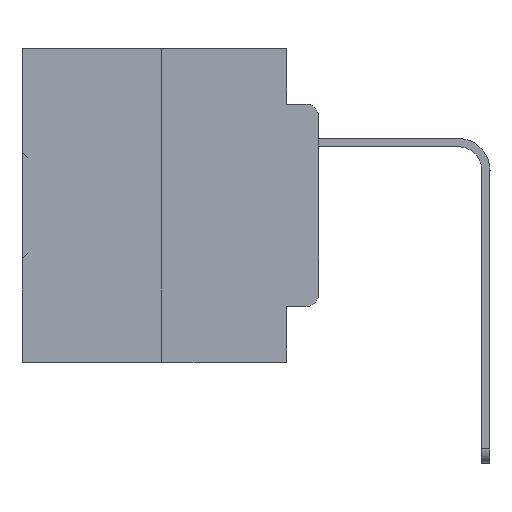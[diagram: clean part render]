
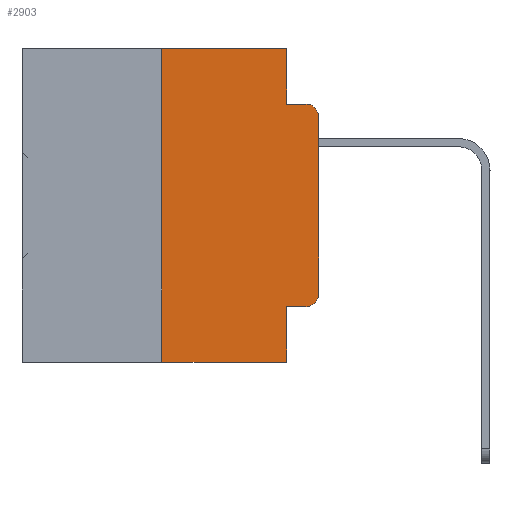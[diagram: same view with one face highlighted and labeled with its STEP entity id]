
A CAD part, left-side view. The second image highlights one B-rep face of the part: STEP entity #2903.
In plain terms, the highlighted planar face has unit normal (-1, 0, 0).
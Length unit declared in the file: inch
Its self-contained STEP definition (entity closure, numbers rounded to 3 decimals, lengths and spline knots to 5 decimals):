
#876 = EDGE_LOOP ( 'NONE', ( #3485, #27984, #14469, #26776, #28233, #36479, #4649, #27697, #25690, #18852 ) ) ;
#1336 = DIRECTION ( 'NONE',  ( 0., 0., -1. ) ) ;
#1850 = CARTESIAN_POINT ( 'NONE',  ( 0., 0.051, -0.4115 ) ) ;
#2461 = EDGE_CURVE ( 'NONE', #5087, #25818, #3342, .T. ) ;
#2837 = DIRECTION ( 'NONE',  ( 0., -1., 0. ) ) ;
#2903 = ADVANCED_FACE ( 'NONE', ( #31973 ), #5675, .F. ) ;
#3047 = DIRECTION ( 'NONE',  ( 0., 0., -1. ) ) ;
#3148 = VERTEX_POINT ( 'NONE', #23831 ) ;
#3251 = CIRCLE ( 'NONE', #27293, 0.02 ) ;
#3342 = LINE ( 'NONE', #25130, #12143 ) ;
#3485 = ORIENTED_EDGE ( 'NONE', *, *, #24115, .T. ) ;
#4204 = DIRECTION ( 'NONE',  ( 0., 0., 1. ) ) ;
#4649 = ORIENTED_EDGE ( 'NONE', *, *, #34257, .T. ) ;
#5087 = VERTEX_POINT ( 'NONE', #1850 ) ;
#5675 = PLANE ( 'NONE',  #17925 ) ;
#6218 = EDGE_CURVE ( 'NONE', #18391, #14889, #28655, .T. ) ;
#6763 = EDGE_CURVE ( 'NONE', #32839, #18391, #25930, .T. ) ;
#7319 = AXIS2_PLACEMENT_3D ( 'NONE', #21485, #21722, #10677 ) ;
#7865 = LINE ( 'NONE', #14119, #29493 ) ;
#9193 = EDGE_CURVE ( 'NONE', #25818, #26109, #3251, .T. ) ;
#9205 = VECTOR ( 'NONE', #1336, 39.37008 ) ;
#9571 = VECTOR ( 'NONE', #4204, 39.37008 ) ;
#9759 = CARTESIAN_POINT ( 'NONE',  ( 0., 0., 0. ) ) ;
#10613 = LINE ( 'NONE', #32290, #28263 ) ;
#10677 = DIRECTION ( 'NONE',  ( 0., 0., -1. ) ) ;
#11140 = CARTESIAN_POINT ( 'NONE',  ( 0., 0.02, -0.4115 ) ) ;
#12143 = VECTOR ( 'NONE', #2837, 39.37008 ) ;
#12409 = EDGE_CURVE ( 'NONE', #31313, #32839, #15794, .T. ) ;
#12755 = EDGE_CURVE ( 'NONE', #17602, #14889, #33425, .T. ) ;
#13996 = CARTESIAN_POINT ( 'NONE',  ( 0., 0.25, -0.5 ) ) ;
#14049 = CARTESIAN_POINT ( 'NONE',  ( 0., 0.473, 0. ) ) ;
#14119 = CARTESIAN_POINT ( 'NONE',  ( 0., 0.473, -0.5 ) ) ;
#14469 = ORIENTED_EDGE ( 'NONE', *, *, #6218, .F. ) ;
#14889 = VERTEX_POINT ( 'NONE', #31507 ) ;
#14898 = VECTOR ( 'NONE', #32012, 39.37008 ) ;
#15393 = CARTESIAN_POINT ( 'NONE',  ( 0., 0.051, 0. ) ) ;
#15545 = CARTESIAN_POINT ( 'NONE',  ( 0., 0.02, -0.3915 ) ) ;
#15794 = LINE ( 'NONE', #33511, #14898 ) ;
#16038 = CARTESIAN_POINT ( 'NONE',  ( 0., 0., -0.1085 ) ) ;
#16586 = DIRECTION ( 'NONE',  ( 0., -1., 0. ) ) ;
#17551 = EDGE_CURVE ( 'NONE', #21590, #31313, #10613, .T. ) ;
#17602 = VERTEX_POINT ( 'NONE', #16038 ) ;
#17925 = AXIS2_PLACEMENT_3D ( 'NONE', #14049, #25697, #3047 ) ;
#18391 = VERTEX_POINT ( 'NONE', #32585 ) ;
#18852 = ORIENTED_EDGE ( 'NONE', *, *, #9193, .T. ) ;
#19684 = LINE ( 'NONE', #9759, #9571 ) ;
#20548 = CARTESIAN_POINT ( 'NONE',  ( 0., 0., -0.3915 ) ) ;
#21032 = DIRECTION ( 'NONE',  ( 0., 0., 1. ) ) ;
#21110 = VECTOR ( 'NONE', #30023, 39.37008 ) ;
#21166 = DIRECTION ( 'NONE',  ( 0., 0., -1. ) ) ;
#21485 = CARTESIAN_POINT ( 'NONE',  ( 0., 0.02, -0.1085 ) ) ;
#21590 = VERTEX_POINT ( 'NONE', #13996 ) ;
#21722 = DIRECTION ( 'NONE',  ( -1., 0., 0. ) ) ;
#22290 = DIRECTION ( 'NONE',  ( 0., 0., -1. ) ) ;
#23765 = DIRECTION ( 'NONE',  ( -1., 0., 0. ) ) ;
#23831 = CARTESIAN_POINT ( 'NONE',  ( 0., 0.051, -0.5 ) ) ;
#24115 = EDGE_CURVE ( 'NONE', #26109, #17602, #19684, .T. ) ;
#25130 = CARTESIAN_POINT ( 'NONE',  ( 0., 0.051, -0.4115 ) ) ;
#25449 = CARTESIAN_POINT ( 'NONE',  ( 0., 0.051, 0. ) ) ;
#25690 = ORIENTED_EDGE ( 'NONE', *, *, #2461, .T. ) ;
#25697 = DIRECTION ( 'NONE',  ( 1., 0., 0. ) ) ;
#25818 = VERTEX_POINT ( 'NONE', #11140 ) ;
#25930 = LINE ( 'NONE', #15393, #9205 ) ;
#26109 = VERTEX_POINT ( 'NONE', #20548 ) ;
#26776 = ORIENTED_EDGE ( 'NONE', *, *, #6763, .F. ) ;
#27293 = AXIS2_PLACEMENT_3D ( 'NONE', #15545, #23765, #21166 ) ;
#27697 = ORIENTED_EDGE ( 'NONE', *, *, #29951, .F. ) ;
#27984 = ORIENTED_EDGE ( 'NONE', *, *, #12755, .T. ) ;
#28233 = ORIENTED_EDGE ( 'NONE', *, *, #12409, .F. ) ;
#28263 = VECTOR ( 'NONE', #21032, 39.37008 ) ;
#28655 = LINE ( 'NONE', #32706, #21110 ) ;
#29493 = VECTOR ( 'NONE', #16586, 39.37008 ) ;
#29951 = EDGE_CURVE ( 'NONE', #5087, #3148, #30265, .T. ) ;
#30023 = DIRECTION ( 'NONE',  ( 0., -1., 0. ) ) ;
#30265 = LINE ( 'NONE', #33540, #33776 ) ;
#31313 = VERTEX_POINT ( 'NONE', #34852 ) ;
#31507 = CARTESIAN_POINT ( 'NONE',  ( 0., 0.02, -0.0885 ) ) ;
#31973 = FACE_OUTER_BOUND ( 'NONE', #876, .T. ) ;
#32012 = DIRECTION ( 'NONE',  ( 0., -1., 0. ) ) ;
#32290 = CARTESIAN_POINT ( 'NONE',  ( 0., 0.25, 0. ) ) ;
#32585 = CARTESIAN_POINT ( 'NONE',  ( 0., 0.051, -0.0885 ) ) ;
#32706 = CARTESIAN_POINT ( 'NONE',  ( 0., 0.051, -0.0885 ) ) ;
#32839 = VERTEX_POINT ( 'NONE', #25449 ) ;
#33425 = CIRCLE ( 'NONE', #7319, 0.02 ) ;
#33511 = CARTESIAN_POINT ( 'NONE',  ( 0., 0.473, 0. ) ) ;
#33540 = CARTESIAN_POINT ( 'NONE',  ( 0., 0.051, 0. ) ) ;
#33776 = VECTOR ( 'NONE', #22290, 39.37008 ) ;
#34257 = EDGE_CURVE ( 'NONE', #21590, #3148, #7865, .T. ) ;
#34852 = CARTESIAN_POINT ( 'NONE',  ( 0., 0.25, 0. ) ) ;
#36479 = ORIENTED_EDGE ( 'NONE', *, *, #17551, .F. ) ;
